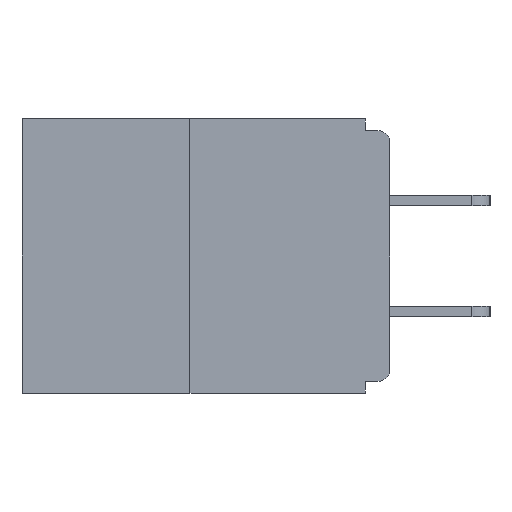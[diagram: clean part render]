
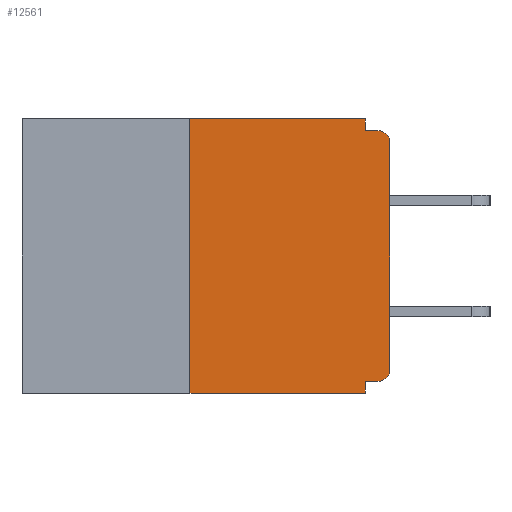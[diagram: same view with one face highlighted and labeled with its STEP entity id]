
A CAD part, left-side view. The second image highlights one B-rep face of the part: STEP entity #12561.
In plain terms, the highlighted planar face has unit normal (-1, 0, 0).
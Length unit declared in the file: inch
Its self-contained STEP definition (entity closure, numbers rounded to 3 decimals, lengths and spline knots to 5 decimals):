
#74 = VECTOR ( 'NONE', #8646, 39.37008 ) ;
#447 = CARTESIAN_POINT ( 'NONE',  ( 0., 0.031, -0.343 ) ) ;
#758 = ORIENTED_EDGE ( 'NONE', *, *, #17728, .F. ) ;
#1320 = DIRECTION ( 'NONE',  ( 0., 0., -1. ) ) ;
#1617 = ORIENTED_EDGE ( 'NONE', *, *, #14882, .F. ) ;
#2018 = DIRECTION ( 'NONE',  ( 0., 0., -1. ) ) ;
#2138 = CARTESIAN_POINT ( 'NONE',  ( 0., 0.015, -0.03 ) ) ;
#2267 = CIRCLE ( 'NONE', #24972, 0.015 ) ;
#2643 = VECTOR ( 'NONE', #19630, 39.37008 ) ;
#2878 = EDGE_CURVE ( 'NONE', #25477, #20082, #17265, .T. ) ;
#3441 = EDGE_CURVE ( 'NONE', #9019, #21492, #23474, .T. ) ;
#3552 = PLANE ( 'NONE',  #9317 ) ;
#4090 = VECTOR ( 'NONE', #24181, 39.37008 ) ;
#5272 = DIRECTION ( 'NONE',  ( 0., 0., 1. ) ) ;
#5513 = EDGE_CURVE ( 'NONE', #9019, #14935, #2267, .T. ) ;
#5795 = LINE ( 'NONE', #12233, #10740 ) ;
#6251 = VECTOR ( 'NONE', #6475, 39.37008 ) ;
#6475 = DIRECTION ( 'NONE',  ( 0., 1., 0. ) ) ;
#6496 = EDGE_CURVE ( 'NONE', #9581, #12396, #10363, .T. ) ;
#6564 = VECTOR ( 'NONE', #5272, 39.37008 ) ;
#7382 = DIRECTION ( 'NONE',  ( -1., 0., 0. ) ) ;
#7597 = VERTEX_POINT ( 'NONE', #447 ) ;
#7606 = VECTOR ( 'NONE', #20017, 39.37008 ) ;
#8646 = DIRECTION ( 'NONE',  ( 0., -1., 0. ) ) ;
#8899 = VERTEX_POINT ( 'NONE', #9091 ) ;
#9019 = VERTEX_POINT ( 'NONE', #16688 ) ;
#9091 = CARTESIAN_POINT ( 'NONE',  ( 0., 0.25, -0.343 ) ) ;
#9317 = AXIS2_PLACEMENT_3D ( 'NONE', #13729, #11492, #1320 ) ;
#9581 = VERTEX_POINT ( 'NONE', #16278 ) ;
#10333 = CARTESIAN_POINT ( 'NONE',  ( 0., 0.031, 0. ) ) ;
#10363 = CIRCLE ( 'NONE', #24609, 0.015 ) ;
#10740 = VECTOR ( 'NONE', #14308, 39.37008 ) ;
#11126 = CARTESIAN_POINT ( 'NONE',  ( 0., 0.031, 0. ) ) ;
#11492 = DIRECTION ( 'NONE',  ( 1., 0., 0. ) ) ;
#11873 = ORIENTED_EDGE ( 'NONE', *, *, #6496, .T. ) ;
#12233 = CARTESIAN_POINT ( 'NONE',  ( 0., 0.46, -0.343 ) ) ;
#12396 = VERTEX_POINT ( 'NONE', #27262 ) ;
#12561 = ADVANCED_FACE ( 'NONE', ( #16248 ), #3552, .F. ) ;
#13478 = LINE ( 'NONE', #21980, #7606 ) ;
#13729 = CARTESIAN_POINT ( 'NONE',  ( 0., 0.46, 0. ) ) ;
#14235 = EDGE_CURVE ( 'NONE', #20082, #12396, #23308, .T. ) ;
#14308 = DIRECTION ( 'NONE',  ( 0., -1., 0. ) ) ;
#14581 = CARTESIAN_POINT ( 'NONE',  ( 0., 0., -0.328 ) ) ;
#14699 = DIRECTION ( 'NONE',  ( -1., 0., 0. ) ) ;
#14882 = EDGE_CURVE ( 'NONE', #21492, #7597, #13478, .T. ) ;
#14935 = VERTEX_POINT ( 'NONE', #23196 ) ;
#15526 = CARTESIAN_POINT ( 'NONE',  ( 0., 0.46, 0. ) ) ;
#15836 = ORIENTED_EDGE ( 'NONE', *, *, #3441, .F. ) ;
#15870 = LINE ( 'NONE', #22016, #6564 ) ;
#15892 = DIRECTION ( 'NONE',  ( 0., 0., -1. ) ) ;
#16248 = FACE_OUTER_BOUND ( 'NONE', #26041, .T. ) ;
#16278 = CARTESIAN_POINT ( 'NONE',  ( 0., 0., -0.03 ) ) ;
#16355 = CARTESIAN_POINT ( 'NONE',  ( 0., 0.25, 0. ) ) ;
#16491 = VERTEX_POINT ( 'NONE', #16355 ) ;
#16688 = CARTESIAN_POINT ( 'NONE',  ( 0., 0.015, -0.328 ) ) ;
#16922 = EDGE_CURVE ( 'NONE', #8899, #16491, #20374, .T. ) ;
#17265 = LINE ( 'NONE', #11126, #2643 ) ;
#17461 = EDGE_CURVE ( 'NONE', #8899, #7597, #5795, .T. ) ;
#17531 = CARTESIAN_POINT ( 'NONE',  ( 0., 0.031, -0.328 ) ) ;
#17728 = EDGE_CURVE ( 'NONE', #16491, #25477, #21534, .T. ) ;
#19499 = ORIENTED_EDGE ( 'NONE', *, *, #17461, .T. ) ;
#19630 = DIRECTION ( 'NONE',  ( 0., 0., -1. ) ) ;
#19942 = DIRECTION ( 'NONE',  ( 0., 0., 1. ) ) ;
#20017 = DIRECTION ( 'NONE',  ( 0., 0., -1. ) ) ;
#20082 = VERTEX_POINT ( 'NONE', #22032 ) ;
#20156 = ORIENTED_EDGE ( 'NONE', *, *, #26479, .T. ) ;
#20374 = LINE ( 'NONE', #26906, #24852 ) ;
#21492 = VERTEX_POINT ( 'NONE', #17531 ) ;
#21534 = LINE ( 'NONE', #15526, #4090 ) ;
#21980 = CARTESIAN_POINT ( 'NONE',  ( 0., 0.031, -0.343 ) ) ;
#22016 = CARTESIAN_POINT ( 'NONE',  ( 0., 0., 0. ) ) ;
#22032 = CARTESIAN_POINT ( 'NONE',  ( 0., 0.031, -0.015 ) ) ;
#23196 = CARTESIAN_POINT ( 'NONE',  ( 0., 0., -0.313 ) ) ;
#23308 = LINE ( 'NONE', #23567, #74 ) ;
#23474 = LINE ( 'NONE', #14581, #6251 ) ;
#23567 = CARTESIAN_POINT ( 'NONE',  ( 0., 0., -0.015 ) ) ;
#23797 = ORIENTED_EDGE ( 'NONE', *, *, #2878, .F. ) ;
#24181 = DIRECTION ( 'NONE',  ( 0., -1., 0. ) ) ;
#24249 = ORIENTED_EDGE ( 'NONE', *, *, #16922, .F. ) ;
#24609 = AXIS2_PLACEMENT_3D ( 'NONE', #2138, #14699, #2018 ) ;
#24852 = VECTOR ( 'NONE', #19942, 39.37008 ) ;
#24972 = AXIS2_PLACEMENT_3D ( 'NONE', #26473, #7382, #15892 ) ;
#25393 = ORIENTED_EDGE ( 'NONE', *, *, #5513, .T. ) ;
#25477 = VERTEX_POINT ( 'NONE', #10333 ) ;
#25759 = ORIENTED_EDGE ( 'NONE', *, *, #14235, .F. ) ;
#26041 = EDGE_LOOP ( 'NONE', ( #758, #24249, #19499, #1617, #15836, #25393, #20156, #11873, #25759, #23797 ) ) ;
#26473 = CARTESIAN_POINT ( 'NONE',  ( 0., 0.015, -0.313 ) ) ;
#26479 = EDGE_CURVE ( 'NONE', #14935, #9581, #15870, .T. ) ;
#26906 = CARTESIAN_POINT ( 'NONE',  ( 0., 0.25, 0. ) ) ;
#27262 = CARTESIAN_POINT ( 'NONE',  ( 0., 0.015, -0.015 ) ) ;
